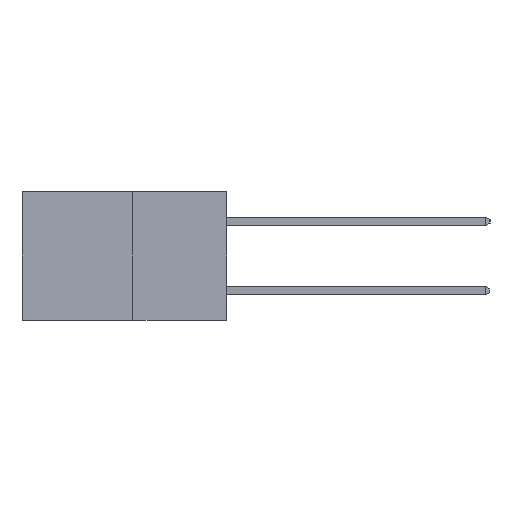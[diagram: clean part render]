
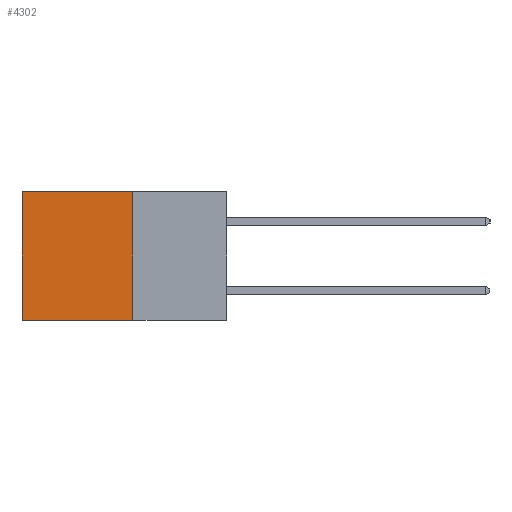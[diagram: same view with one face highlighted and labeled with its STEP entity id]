
A CAD part, left-side view. The second image highlights one B-rep face of the part: STEP entity #4302.
In plain terms, the highlighted planar face has unit normal (-1, 0, 0).
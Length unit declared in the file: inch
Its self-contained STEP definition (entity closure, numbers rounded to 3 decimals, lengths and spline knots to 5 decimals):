
#1007 = CARTESIAN_POINT ( 'NONE',  ( 0.277, 0.59, -0.37 ) ) ;
#1065 = CARTESIAN_POINT ( 'NONE',  ( 0.277, 0.27, 0. ) ) ;
#1559 = VERTEX_POINT ( 'NONE', #7608 ) ;
#1865 = CARTESIAN_POINT ( 'NONE',  ( 0.277, 0.27, -0.37 ) ) ;
#2037 = EDGE_CURVE ( 'NONE', #8717, #2716, #6215, .T. ) ;
#2234 = EDGE_CURVE ( 'NONE', #2716, #1559, #2328, .T. ) ;
#2328 = LINE ( 'NONE', #1007, #6667 ) ;
#2474 = CARTESIAN_POINT ( 'NONE',  ( 0.277, 0.27, -0.37 ) ) ;
#2716 = VERTEX_POINT ( 'NONE', #4452 ) ;
#2752 = CARTESIAN_POINT ( 'NONE',  ( 0.277, 0.27, -0.37 ) ) ;
#2909 = PLANE ( 'NONE',  #5498 ) ;
#3024 = VECTOR ( 'NONE', #3724, 39.37008 ) ;
#3076 = ORIENTED_EDGE ( 'NONE', *, *, #2234, .T. ) ;
#3289 = VECTOR ( 'NONE', #4102, 39.37008 ) ;
#3536 = DIRECTION ( 'NONE',  ( 0., 0., -1. ) ) ;
#3593 = DIRECTION ( 'NONE',  ( 1., 0., 0. ) ) ;
#3640 = CARTESIAN_POINT ( 'NONE',  ( 0.277, 0.27, -0.37 ) ) ;
#3724 = DIRECTION ( 'NONE',  ( 0., 0., -1. ) ) ;
#4073 = EDGE_CURVE ( 'NONE', #4620, #1559, #8285, .T. ) ;
#4102 = DIRECTION ( 'NONE',  ( 0., 1., 0. ) ) ;
#4302 = ADVANCED_FACE ( 'NONE', ( #8723 ), #2909, .F. ) ;
#4452 = CARTESIAN_POINT ( 'NONE',  ( 0.277, 0.59, 0. ) ) ;
#4478 = EDGE_CURVE ( 'NONE', #8717, #4620, #6250, .T. ) ;
#4549 = VECTOR ( 'NONE', #5895, 39.37008 ) ;
#4620 = VERTEX_POINT ( 'NONE', #1865 ) ;
#5498 = AXIS2_PLACEMENT_3D ( 'NONE', #2752, #3593, #3536 ) ;
#5895 = DIRECTION ( 'NONE',  ( 0., 1., 0. ) ) ;
#6213 = ORIENTED_EDGE ( 'NONE', *, *, #4073, .F. ) ;
#6215 = LINE ( 'NONE', #6914, #4549 ) ;
#6250 = LINE ( 'NONE', #3640, #3024 ) ;
#6332 = ORIENTED_EDGE ( 'NONE', *, *, #2037, .T. ) ;
#6367 = ORIENTED_EDGE ( 'NONE', *, *, #4478, .F. ) ;
#6667 = VECTOR ( 'NONE', #6856, 39.37008 ) ;
#6856 = DIRECTION ( 'NONE',  ( 0., 0., -1. ) ) ;
#6914 = CARTESIAN_POINT ( 'NONE',  ( 0.277, 0.27, 0. ) ) ;
#7284 = EDGE_LOOP ( 'NONE', ( #3076, #6213, #6367, #6332 ) ) ;
#7608 = CARTESIAN_POINT ( 'NONE',  ( 0.277, 0.59, -0.37 ) ) ;
#8285 = LINE ( 'NONE', #2474, #3289 ) ;
#8717 = VERTEX_POINT ( 'NONE', #1065 ) ;
#8723 = FACE_OUTER_BOUND ( 'NONE', #7284, .T. ) ;
